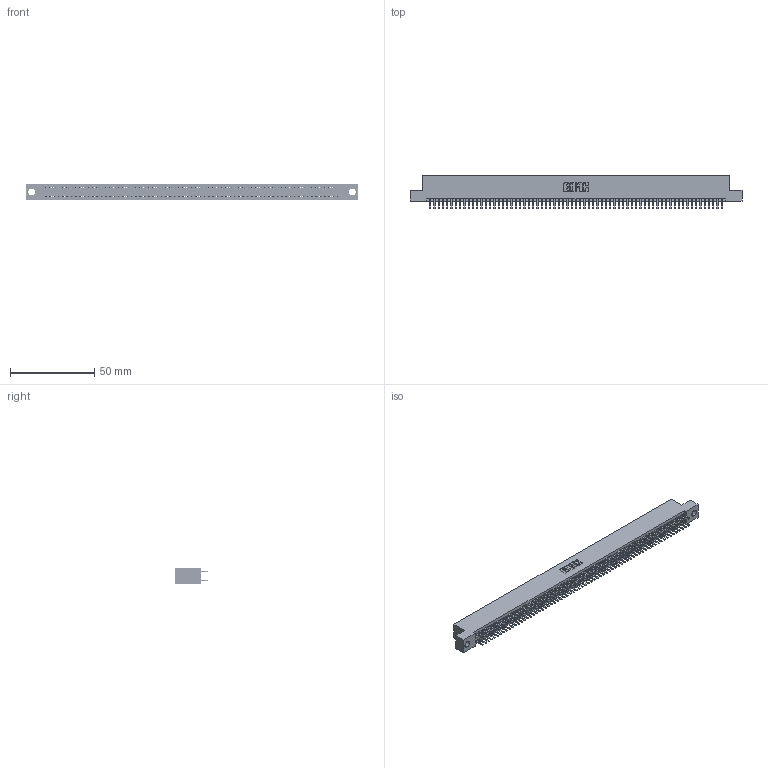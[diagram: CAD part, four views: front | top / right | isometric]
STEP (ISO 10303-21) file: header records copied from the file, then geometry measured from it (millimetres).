
FILE_DESCRIPTION (( 'STEP AP203' ), '1' );
FILE_NAME ('345-138-520-204.STEP', '2018-10-20T17:02:55', ( '' ), ( '' ), 'SwSTEP 2.0', 'SolidWorks 2016', '' );
FILE_SCHEMA (( 'CONFIG_CONTROL_DESIGN' ));
Length unit declared in the file: inch
Products named in the file (3): 345-292-001_345-293-120; 345-138-520-204; 345 Part_Flush Mounting Lugs - 0.156 Dia-TH
Assembly tree (139 placements, depth 2):
  345-138-520-204
    345 Part_Flush Mounting Lugs - 0.156 Dia-TH
    345-292-001_345-293-120  x138
Bounding box: 196.47 x 19.68 x 9.4 mm (x, y, z)
Volume: 19187.3 mm3; surface area: 28571.1 mm2
Topology: 139 solids, 139 shells, 7578 faces, 22007 edges, 14302 vertices
Faces by surface type: plane 4910, cylinder 2668
Entity records: 50621 total; most frequent: CARTESIAN_POINT 8472, ORIENTED_EDGE 8394, DIRECTION 7425, EDGE_CURVE 4197, LINE 3785, VECTOR 3785, VERTEX_POINT 2794, AXIS2_PLACEMENT_3D 1820
